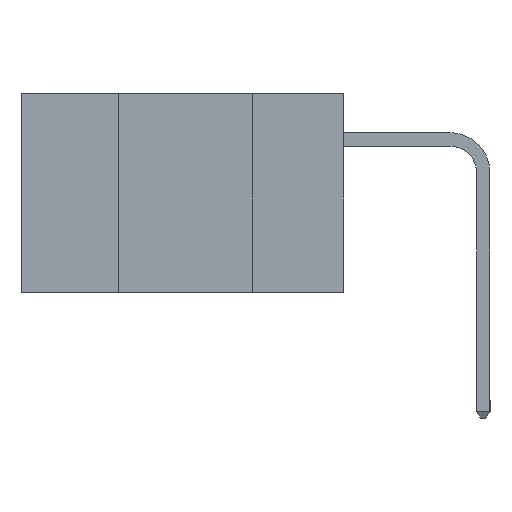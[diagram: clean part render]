
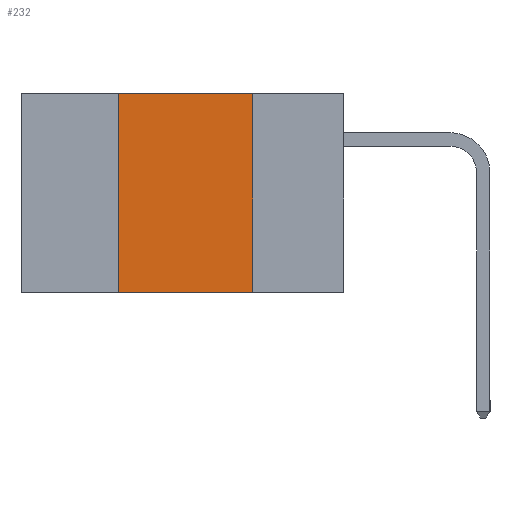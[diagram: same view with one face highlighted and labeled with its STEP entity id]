
A CAD part, left-side view. The second image highlights one B-rep face of the part: STEP entity #232.
In plain terms, the highlighted planar face has unit normal (-1, 0, 0).
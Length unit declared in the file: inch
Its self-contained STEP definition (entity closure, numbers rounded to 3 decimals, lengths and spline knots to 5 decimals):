
#3 = EDGE_LOOP ( 'NONE', ( #4667, #235, #8337, #4415 ) ) ;
#215 = FACE_OUTER_BOUND ( 'NONE', #3, .T. ) ;
#232 = ADVANCED_FACE ( 'NONE', ( #215 ), #3063, .F. ) ;
#235 = ORIENTED_EDGE ( 'NONE', *, *, #8623, .F. ) ;
#479 = DIRECTION ( 'NONE',  ( 0., 0., 1. ) ) ;
#791 = LINE ( 'NONE', #1366, #8316 ) ;
#918 = CARTESIAN_POINT ( 'NONE',  ( 0., 0.42, -0.37 ) ) ;
#953 = DIRECTION ( 'NONE',  ( 0., -1., 0. ) ) ;
#1078 = VERTEX_POINT ( 'NONE', #918 ) ;
#1366 = CARTESIAN_POINT ( 'NONE',  ( 0., 0.17, -0.37 ) ) ;
#1677 = LINE ( 'NONE', #2657, #5655 ) ;
#2155 = DIRECTION ( 'NONE',  ( 0., 0., -1. ) ) ;
#2513 = VERTEX_POINT ( 'NONE', #8568 ) ;
#2657 = CARTESIAN_POINT ( 'NONE',  ( 0., 0.6, 0. ) ) ;
#2832 = CARTESIAN_POINT ( 'NONE',  ( 0., 0.6, -0.37 ) ) ;
#2881 = CARTESIAN_POINT ( 'NONE',  ( 0., 0.42, -0.37 ) ) ;
#2955 = EDGE_CURVE ( 'NONE', #1078, #2513, #9218, .T. ) ;
#3016 = VECTOR ( 'NONE', #953, 39.37008 ) ;
#3063 = PLANE ( 'NONE',  #9941 ) ;
#3068 = EDGE_CURVE ( 'NONE', #1078, #6983, #3929, .T. ) ;
#3453 = CARTESIAN_POINT ( 'NONE',  ( 0., 0.42, 0. ) ) ;
#3465 = DIRECTION ( 'NONE',  ( 0., -1., 0. ) ) ;
#3665 = VECTOR ( 'NONE', #479, 39.37008 ) ;
#3929 = LINE ( 'NONE', #2881, #3665 ) ;
#4256 = CARTESIAN_POINT ( 'NONE',  ( 0., 0.6, 0. ) ) ;
#4415 = ORIENTED_EDGE ( 'NONE', *, *, #2955, .T. ) ;
#4519 = DIRECTION ( 'NONE',  ( 1., 0., 0. ) ) ;
#4667 = ORIENTED_EDGE ( 'NONE', *, *, #9574, .F. ) ;
#5655 = VECTOR ( 'NONE', #3465, 39.37008 ) ;
#6983 = VERTEX_POINT ( 'NONE', #3453 ) ;
#8316 = VECTOR ( 'NONE', #2155, 39.37008 ) ;
#8326 = VERTEX_POINT ( 'NONE', #9846 ) ;
#8337 = ORIENTED_EDGE ( 'NONE', *, *, #3068, .F. ) ;
#8568 = CARTESIAN_POINT ( 'NONE',  ( 0., 0.17, -0.37 ) ) ;
#8623 = EDGE_CURVE ( 'NONE', #6983, #8326, #1677, .T. ) ;
#9218 = LINE ( 'NONE', #2832, #3016 ) ;
#9574 = EDGE_CURVE ( 'NONE', #8326, #2513, #791, .T. ) ;
#9690 = DIRECTION ( 'NONE',  ( 0., 0., -1. ) ) ;
#9846 = CARTESIAN_POINT ( 'NONE',  ( 0., 0.17, 0. ) ) ;
#9941 = AXIS2_PLACEMENT_3D ( 'NONE', #4256, #4519, #9690 ) ;
